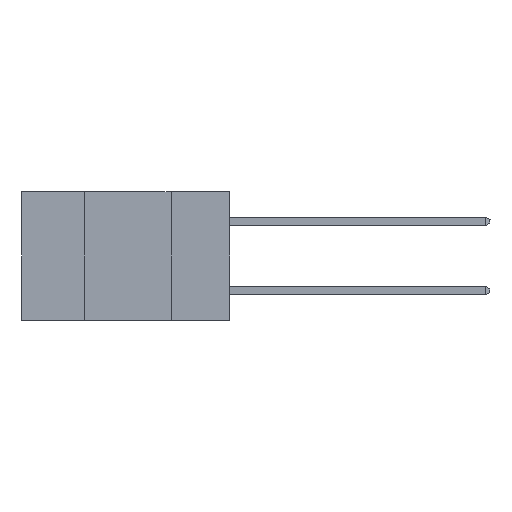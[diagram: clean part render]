
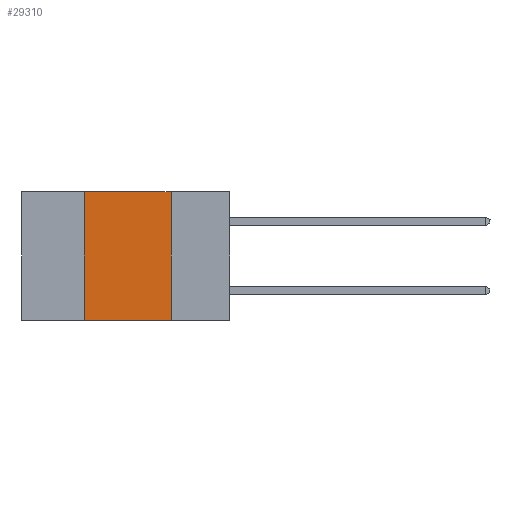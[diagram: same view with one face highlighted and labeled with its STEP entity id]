
A CAD part, left-side view. The second image highlights one B-rep face of the part: STEP entity #29310.
In plain terms, the highlighted planar face has unit normal (-1, 0, 0).
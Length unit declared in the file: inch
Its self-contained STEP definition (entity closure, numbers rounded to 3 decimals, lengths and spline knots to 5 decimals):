
#504 = CARTESIAN_POINT ( 'NONE',  ( 0., 0.42, -0.37 ) ) ;
#1219 = DIRECTION ( 'NONE',  ( 0., -1., 0. ) ) ;
#1579 = VERTEX_POINT ( 'NONE', #25201 ) ;
#2686 = CARTESIAN_POINT ( 'NONE',  ( 0., 0.6, 0. ) ) ;
#3710 = DIRECTION ( 'NONE',  ( 0., 0., -1. ) ) ;
#4172 = VECTOR ( 'NONE', #27408, 39.37008 ) ;
#4194 = VECTOR ( 'NONE', #31188, 39.37008 ) ;
#5954 = ORIENTED_EDGE ( 'NONE', *, *, #6866, .F. ) ;
#6866 = EDGE_CURVE ( 'NONE', #25634, #27491, #16640, .T. ) ;
#7081 = ORIENTED_EDGE ( 'NONE', *, *, #22060, .F. ) ;
#7218 = DIRECTION ( 'NONE',  ( 0., 0., -1. ) ) ;
#7897 = CARTESIAN_POINT ( 'NONE',  ( 0., 0.42, 0. ) ) ;
#8727 = CARTESIAN_POINT ( 'NONE',  ( 0., 0.6, -0.37 ) ) ;
#11295 = LINE ( 'NONE', #19648, #29500 ) ;
#12165 = ORIENTED_EDGE ( 'NONE', *, *, #17639, .F. ) ;
#15556 = VECTOR ( 'NONE', #1219, 39.37008 ) ;
#15894 = FACE_OUTER_BOUND ( 'NONE', #26614, .T. ) ;
#16640 = LINE ( 'NONE', #30369, #4194 ) ;
#17543 = VERTEX_POINT ( 'NONE', #32055 ) ;
#17639 = EDGE_CURVE ( 'NONE', #27491, #17543, #30556, .T. ) ;
#18587 = DIRECTION ( 'NONE',  ( 1., 0., 0. ) ) ;
#19648 = CARTESIAN_POINT ( 'NONE',  ( 0., 0.17, 0. ) ) ;
#20981 = PLANE ( 'NONE',  #24757 ) ;
#22060 = EDGE_CURVE ( 'NONE', #17543, #1579, #11295, .T. ) ;
#24757 = AXIS2_PLACEMENT_3D ( 'NONE', #30894, #18587, #3710 ) ;
#24861 = ORIENTED_EDGE ( 'NONE', *, *, #28650, .T. ) ;
#25201 = CARTESIAN_POINT ( 'NONE',  ( 0., 0.17, -0.37 ) ) ;
#25634 = VERTEX_POINT ( 'NONE', #504 ) ;
#26614 = EDGE_LOOP ( 'NONE', ( #7081, #12165, #5954, #24861 ) ) ;
#27408 = DIRECTION ( 'NONE',  ( 0., -1., 0. ) ) ;
#27491 = VERTEX_POINT ( 'NONE', #7897 ) ;
#27937 = LINE ( 'NONE', #8727, #15556 ) ;
#28650 = EDGE_CURVE ( 'NONE', #25634, #1579, #27937, .T. ) ;
#29310 = ADVANCED_FACE ( 'NONE', ( #15894 ), #20981, .F. ) ;
#29500 = VECTOR ( 'NONE', #7218, 39.37008 ) ;
#30369 = CARTESIAN_POINT ( 'NONE',  ( 0., 0.42, 0. ) ) ;
#30556 = LINE ( 'NONE', #2686, #4172 ) ;
#30894 = CARTESIAN_POINT ( 'NONE',  ( 0., 0.6, 0. ) ) ;
#31188 = DIRECTION ( 'NONE',  ( 0., 0., 1. ) ) ;
#32055 = CARTESIAN_POINT ( 'NONE',  ( 0., 0.17, 0. ) ) ;
